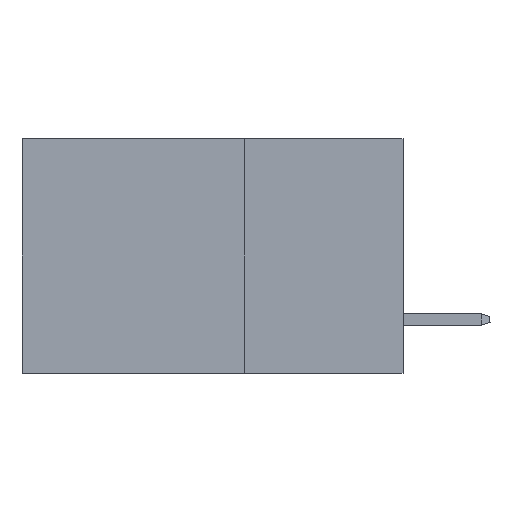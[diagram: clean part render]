
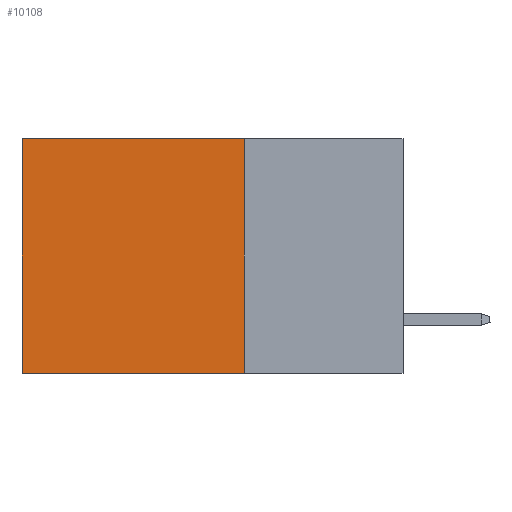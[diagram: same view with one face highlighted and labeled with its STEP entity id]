
A CAD part, left-side view. The second image highlights one B-rep face of the part: STEP entity #10108.
In plain terms, the highlighted planar face has unit normal (-1, 0, 0).
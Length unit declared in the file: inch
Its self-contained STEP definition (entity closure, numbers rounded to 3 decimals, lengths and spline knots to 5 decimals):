
#1459 = CARTESIAN_POINT ( 'NONE',  ( 0.2875, 0.6, -0.37 ) ) ;
#2271 = VERTEX_POINT ( 'NONE', #35109 ) ;
#3322 = LINE ( 'NONE', #22452, #30952 ) ;
#3871 = ORIENTED_EDGE ( 'NONE', *, *, #15503, .F. ) ;
#3960 = VERTEX_POINT ( 'NONE', #10098 ) ;
#4407 = LINE ( 'NONE', #15310, #21563 ) ;
#4644 = VECTOR ( 'NONE', #25183, 39.37008 ) ;
#5320 = CARTESIAN_POINT ( 'NONE',  ( 0.2875, 0.25, 0. ) ) ;
#5450 = DIRECTION ( 'NONE',  ( 0., 1., 0. ) ) ;
#7019 = EDGE_CURVE ( 'NONE', #3960, #2271, #21901, .T. ) ;
#9875 = EDGE_CURVE ( 'NONE', #3960, #19225, #19987, .T. ) ;
#10098 = CARTESIAN_POINT ( 'NONE',  ( 0.2875, 0.25, 0. ) ) ;
#10108 = ADVANCED_FACE ( 'NONE', ( #21945 ), #22293, .F. ) ;
#10813 = VECTOR ( 'NONE', #32813, 39.37008 ) ;
#12227 = ORIENTED_EDGE ( 'NONE', *, *, #9875, .F. ) ;
#13895 = VERTEX_POINT ( 'NONE', #1459 ) ;
#15310 = CARTESIAN_POINT ( 'NONE',  ( 0.2875, 0.25, -0.37 ) ) ;
#15503 = EDGE_CURVE ( 'NONE', #19225, #13895, #4407, .T. ) ;
#19225 = VERTEX_POINT ( 'NONE', #23751 ) ;
#19540 = CARTESIAN_POINT ( 'NONE',  ( 0.2875, 0.25, 0. ) ) ;
#19987 = LINE ( 'NONE', #28398, #4644 ) ;
#20296 = EDGE_LOOP ( 'NONE', ( #30066, #3871, #12227, #28393 ) ) ;
#21563 = VECTOR ( 'NONE', #5450, 39.37008 ) ;
#21901 = LINE ( 'NONE', #19540, #10813 ) ;
#21945 = FACE_OUTER_BOUND ( 'NONE', #20296, .T. ) ;
#22293 = PLANE ( 'NONE',  #32232 ) ;
#22452 = CARTESIAN_POINT ( 'NONE',  ( 0.2875, 0.6, 0. ) ) ;
#23751 = CARTESIAN_POINT ( 'NONE',  ( 0.2875, 0.25, -0.37 ) ) ;
#25183 = DIRECTION ( 'NONE',  ( 0., 0., -1. ) ) ;
#25646 = DIRECTION ( 'NONE',  ( 0., 0., -1. ) ) ;
#26824 = EDGE_CURVE ( 'NONE', #2271, #13895, #3322, .T. ) ;
#27478 = DIRECTION ( 'NONE',  ( 1., 0., 0. ) ) ;
#28393 = ORIENTED_EDGE ( 'NONE', *, *, #7019, .T. ) ;
#28398 = CARTESIAN_POINT ( 'NONE',  ( 0.2875, 0.25, 0. ) ) ;
#29653 = DIRECTION ( 'NONE',  ( 0., 0., -1. ) ) ;
#30066 = ORIENTED_EDGE ( 'NONE', *, *, #26824, .T. ) ;
#30952 = VECTOR ( 'NONE', #25646, 39.37008 ) ;
#32232 = AXIS2_PLACEMENT_3D ( 'NONE', #5320, #27478, #29653 ) ;
#32813 = DIRECTION ( 'NONE',  ( 0., 1., 0. ) ) ;
#35109 = CARTESIAN_POINT ( 'NONE',  ( 0.2875, 0.6, 0. ) ) ;
